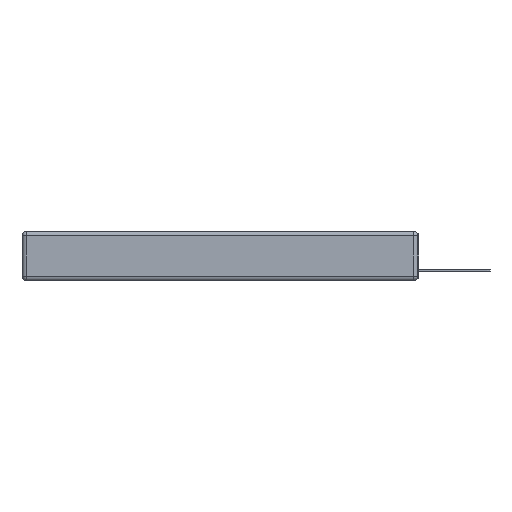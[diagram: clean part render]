
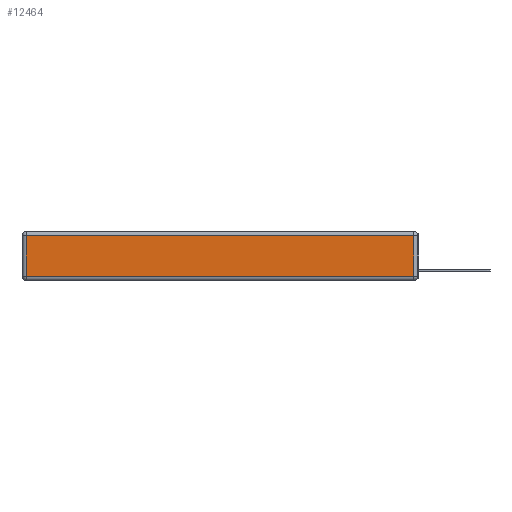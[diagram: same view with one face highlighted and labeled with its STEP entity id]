
A CAD part, left-side view. The second image highlights one B-rep face of the part: STEP entity #12464.
In plain terms, the highlighted planar face has unit normal (-1, 0, 0).
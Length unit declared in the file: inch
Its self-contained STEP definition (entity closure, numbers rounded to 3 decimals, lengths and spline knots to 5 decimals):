
#718 = CARTESIAN_POINT ( 'NONE',  ( 0., 0., -0.343 ) ) ;
#2156 = CARTESIAN_POINT ( 'NONE',  ( 0., 2.72, -0.03 ) ) ;
#2523 = DIRECTION ( 'NONE',  ( -1., 0., 0. ) ) ;
#3240 = VECTOR ( 'NONE', #17801, 39.37008 ) ;
#3772 = LINE ( 'NONE', #22481, #17566 ) ;
#4179 = ORIENTED_EDGE ( 'NONE', *, *, #14230, .T. ) ;
#4220 = EDGE_CURVE ( 'NONE', #14029, #13791, #14664, .T. ) ;
#4237 = ORIENTED_EDGE ( 'NONE', *, *, #4220, .T. ) ;
#4749 = VERTEX_POINT ( 'NONE', #12964 ) ;
#5218 = CARTESIAN_POINT ( 'NONE',  ( 0., 2.72, -0.313 ) ) ;
#6086 = ORIENTED_EDGE ( 'NONE', *, *, #21204, .T. ) ;
#6602 = VERTEX_POINT ( 'NONE', #21476 ) ;
#6607 = EDGE_LOOP ( 'NONE', ( #16717, #6086, #4179, #4237 ) ) ;
#7500 = VECTOR ( 'NONE', #17427, 39.37008 ) ;
#8273 = DIRECTION ( 'NONE',  ( 0., 1., 0. ) ) ;
#8954 = EDGE_CURVE ( 'NONE', #13791, #4749, #17595, .T. ) ;
#11031 = VECTOR ( 'NONE', #22975, 39.37008 ) ;
#11168 = DIRECTION ( 'NONE',  ( 0., 0., 1. ) ) ;
#12049 = CARTESIAN_POINT ( 'NONE',  ( 0., 0.03, -0.343 ) ) ;
#12464 = ADVANCED_FACE ( 'NONE', ( #13580 ), #18593, .T. ) ;
#12964 = CARTESIAN_POINT ( 'NONE',  ( 0., 0.03, -0.313 ) ) ;
#13413 = LINE ( 'NONE', #12049, #7500 ) ;
#13580 = FACE_OUTER_BOUND ( 'NONE', #6607, .T. ) ;
#13791 = VERTEX_POINT ( 'NONE', #5218 ) ;
#14029 = VERTEX_POINT ( 'NONE', #2156 ) ;
#14230 = EDGE_CURVE ( 'NONE', #6602, #14029, #3772, .T. ) ;
#14664 = LINE ( 'NONE', #21468, #11031 ) ;
#16717 = ORIENTED_EDGE ( 'NONE', *, *, #8954, .T. ) ;
#17427 = DIRECTION ( 'NONE',  ( 0., 0., 1. ) ) ;
#17566 = VECTOR ( 'NONE', #8273, 39.37008 ) ;
#17595 = LINE ( 'NONE', #21439, #3240 ) ;
#17801 = DIRECTION ( 'NONE',  ( 0., -1., 0. ) ) ;
#18593 = PLANE ( 'NONE',  #19085 ) ;
#19085 = AXIS2_PLACEMENT_3D ( 'NONE', #718, #2523, #11168 ) ;
#21204 = EDGE_CURVE ( 'NONE', #4749, #6602, #13413, .T. ) ;
#21439 = CARTESIAN_POINT ( 'NONE',  ( 0., 0., -0.313 ) ) ;
#21468 = CARTESIAN_POINT ( 'NONE',  ( 0., 2.72, -0.343 ) ) ;
#21476 = CARTESIAN_POINT ( 'NONE',  ( 0., 0.03, -0.03 ) ) ;
#22481 = CARTESIAN_POINT ( 'NONE',  ( 0., 2.75, -0.03 ) ) ;
#22975 = DIRECTION ( 'NONE',  ( 0., 0., -1. ) ) ;
